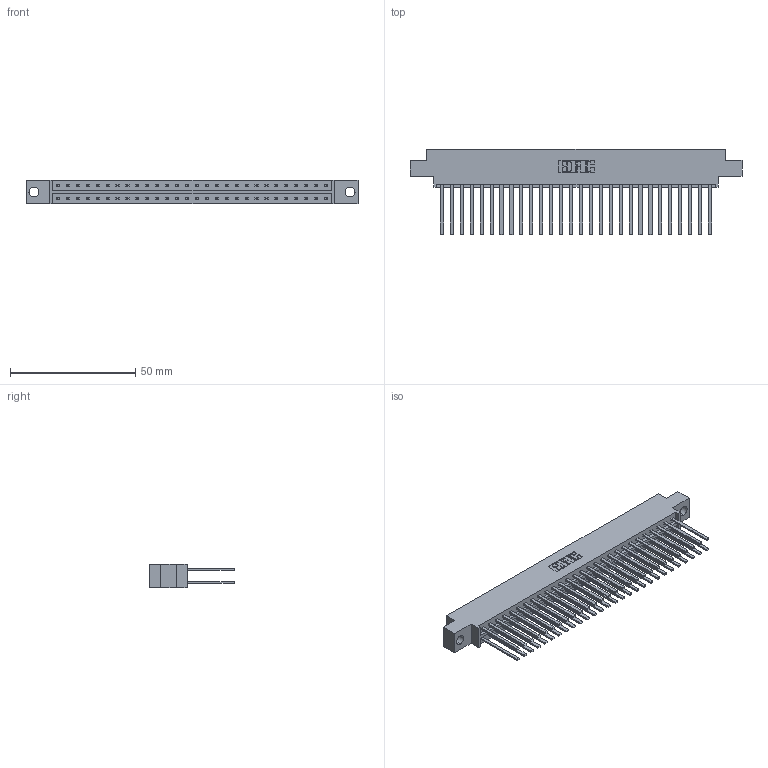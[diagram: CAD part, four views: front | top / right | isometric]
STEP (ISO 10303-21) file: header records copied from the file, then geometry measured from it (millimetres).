
FILE_DESCRIPTION (( 'STEP AP203' ), '1' );
FILE_NAME ('833-056-544-804.STEP', '2020-06-04T23:05:48', ( '' ), ( '' ), 'SwSTEP 2.0', 'SolidWorks 2020', '' );
FILE_SCHEMA (( 'CONFIG_CONTROL_DESIGN' ));
Length unit declared in the file: inch
Products named in the file (3): 345-292-001_345-293-144; 833 Part_Offset - .156 Dia - TH; 833-056-544-804
Assembly tree (57 placements, depth 2):
  833-056-544-804
    833 Part_Offset - .156 Dia - TH
    345-292-001_345-293-144  x56
Bounding box: 132.49 x 34.3 x 9.4 mm (x, y, z)
Volume: 13864.5 mm3; surface area: 18788.7 mm2
Topology: 57 solids, 57 shells, 2694 faces, 7995 edges, 5254 vertices
Faces by surface type: plane 1866, cylinder 828
Entity records: 19775 total; most frequent: CARTESIAN_POINT 3294, ORIENTED_EDGE 3230, DIRECTION 2835, EDGE_CURVE 1615, VECTOR 1491, LINE 1491, VERTEX_POINT 1074, AXIS2_PLACEMENT_3D 672
